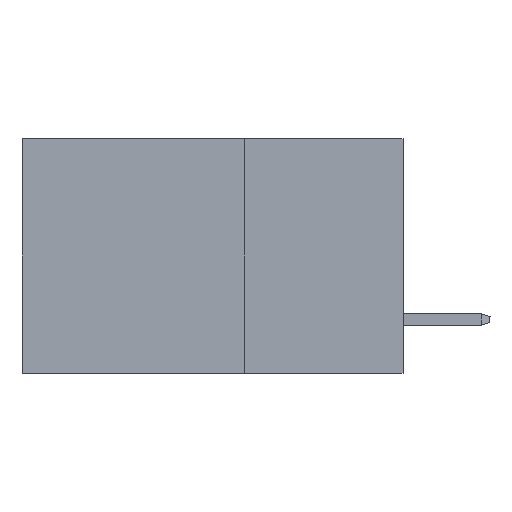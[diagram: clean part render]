
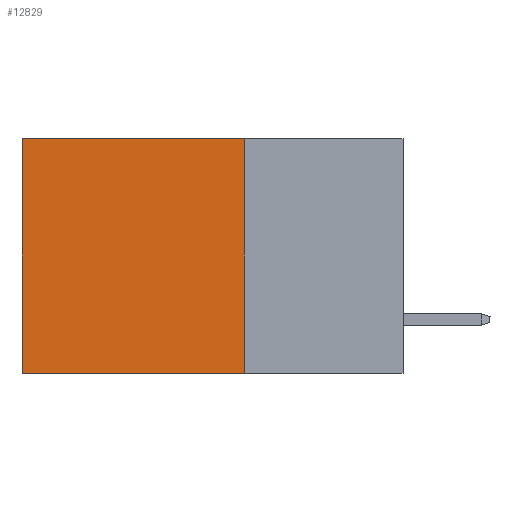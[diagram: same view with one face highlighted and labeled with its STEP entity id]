
A CAD part, left-side view. The second image highlights one B-rep face of the part: STEP entity #12829.
In plain terms, the highlighted planar face has unit normal (-1, 0, 0).
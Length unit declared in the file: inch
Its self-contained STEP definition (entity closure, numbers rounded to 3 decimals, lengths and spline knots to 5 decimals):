
#755 = VERTEX_POINT ( 'NONE', #11985 ) ;
#1334 = LINE ( 'NONE', #25986, #3959 ) ;
#1404 = CARTESIAN_POINT ( 'NONE',  ( 0.2875, 0.25, 0. ) ) ;
#3103 = DIRECTION ( 'NONE',  ( 0., 0., -1. ) ) ;
#3584 = LINE ( 'NONE', #17187, #28478 ) ;
#3959 = VECTOR ( 'NONE', #8132, 39.37008 ) ;
#5319 = DIRECTION ( 'NONE',  ( 1., 0., 0. ) ) ;
#5494 = CARTESIAN_POINT ( 'NONE',  ( 0.2875, 0.6, 0. ) ) ;
#6064 = ORIENTED_EDGE ( 'NONE', *, *, #19687, .T. ) ;
#6259 = DIRECTION ( 'NONE',  ( 0., 1., 0. ) ) ;
#6980 = EDGE_CURVE ( 'NONE', #16592, #25626, #1334, .T. ) ;
#8132 = DIRECTION ( 'NONE',  ( 0., 1., 0. ) ) ;
#8591 = CARTESIAN_POINT ( 'NONE',  ( 0.2875, 0.25, 0. ) ) ;
#10109 = DIRECTION ( 'NONE',  ( 0., 0., -1. ) ) ;
#10152 = VECTOR ( 'NONE', #6259, 39.37008 ) ;
#11633 = ORIENTED_EDGE ( 'NONE', *, *, #17016, .T. ) ;
#11985 = CARTESIAN_POINT ( 'NONE',  ( 0.2875, 0.25, 0. ) ) ;
#12123 = CARTESIAN_POINT ( 'NONE',  ( 0.2875, 0.6, -0.37 ) ) ;
#12426 = LINE ( 'NONE', #8591, #28204 ) ;
#12829 = ADVANCED_FACE ( 'NONE', ( #27753 ), #20965, .F. ) ;
#13066 = LINE ( 'NONE', #1404, #10152 ) ;
#13082 = ORIENTED_EDGE ( 'NONE', *, *, #14074, .F. ) ;
#14074 = EDGE_CURVE ( 'NONE', #755, #16592, #12426, .T. ) ;
#15639 = EDGE_LOOP ( 'NONE', ( #11633, #23880, #13082, #6064 ) ) ;
#16592 = VERTEX_POINT ( 'NONE', #26505 ) ;
#17016 = EDGE_CURVE ( 'NONE', #23953, #25626, #3584, .T. ) ;
#17187 = CARTESIAN_POINT ( 'NONE',  ( 0.2875, 0.6, 0. ) ) ;
#18775 = CARTESIAN_POINT ( 'NONE',  ( 0.2875, 0.25, 0. ) ) ;
#19687 = EDGE_CURVE ( 'NONE', #755, #23953, #13066, .T. ) ;
#20965 = PLANE ( 'NONE',  #23019 ) ;
#23019 = AXIS2_PLACEMENT_3D ( 'NONE', #18775, #5319, #3103 ) ;
#23880 = ORIENTED_EDGE ( 'NONE', *, *, #6980, .F. ) ;
#23953 = VERTEX_POINT ( 'NONE', #5494 ) ;
#25626 = VERTEX_POINT ( 'NONE', #12123 ) ;
#25986 = CARTESIAN_POINT ( 'NONE',  ( 0.2875, 0.25, -0.37 ) ) ;
#26505 = CARTESIAN_POINT ( 'NONE',  ( 0.2875, 0.25, -0.37 ) ) ;
#27753 = FACE_OUTER_BOUND ( 'NONE', #15639, .T. ) ;
#28204 = VECTOR ( 'NONE', #28366, 39.37008 ) ;
#28366 = DIRECTION ( 'NONE',  ( 0., 0., -1. ) ) ;
#28478 = VECTOR ( 'NONE', #10109, 39.37008 ) ;
